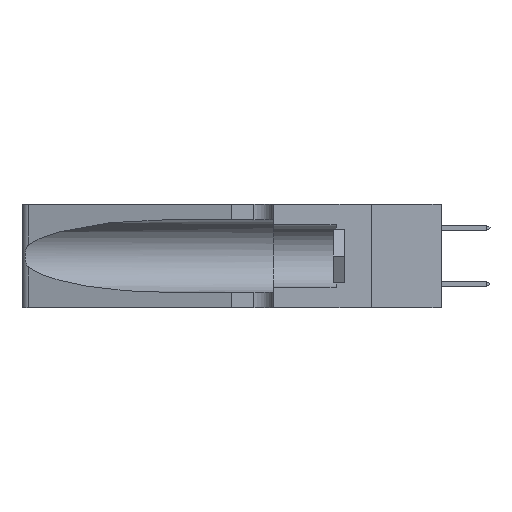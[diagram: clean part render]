
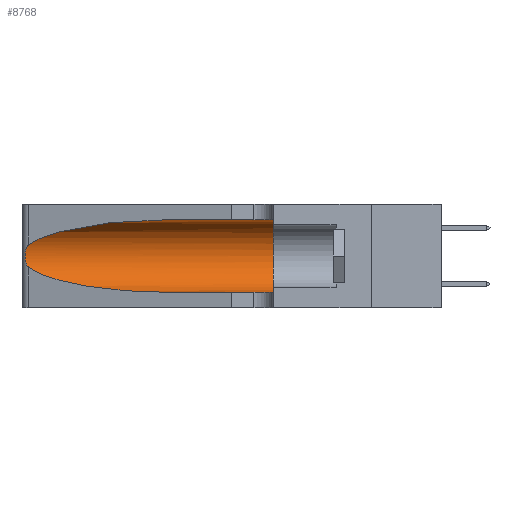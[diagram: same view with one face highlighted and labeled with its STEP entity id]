
A CAD part, left-side view. The second image highlights one B-rep face of the part: STEP entity #8768.
In plain terms, the highlighted cylindrical face has radius 3.308 mm (diameter 6.617 mm), a partial arc.
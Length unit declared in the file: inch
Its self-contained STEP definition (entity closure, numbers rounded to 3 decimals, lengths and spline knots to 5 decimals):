
#13 = LINE ( 'NONE', #13438, #5790 ) ;
#63 = ORIENTED_EDGE ( 'NONE', *, *, #6949, .F. ) ;
#84 =( BOUNDED_CURVE ( )  B_SPLINE_CURVE ( 3, ( #18097, #10203, #13347, #18655 ),
 .UNSPECIFIED., .F., .T. ) 
 B_SPLINE_CURVE_WITH_KNOTS ( ( 4, 4 ),
 ( 1.5708, 2.84003 ),
 .UNSPECIFIED. ) 
 CURVE ( )  GEOMETRIC_REPRESENTATION_ITEM ( )  RATIONAL_B_SPLINE_CURVE ( ( 1., 0.87, 0.87, 1. ) ) 
 REPRESENTATION_ITEM ( '' )  );
#110 = LINE ( 'NONE', #16641, #18577 ) ;
#367 = CARTESIAN_POINT ( 'NONE',  ( 0.25856, 1.23593, 0.16098 ) ) ;
#530 = DIRECTION ( 'NONE',  ( 0., -1., 0. ) ) ;
#2295 = ORIENTED_EDGE ( 'NONE', *, *, #19413, .F. ) ;
#2469 = DIRECTION ( 'NONE',  ( 0., 1., 0. ) ) ;
#3046 = CARTESIAN_POINT ( 'NONE',  ( 0.1305, 0.35, 0.31525 ) ) ;
#3513 = CARTESIAN_POINT ( 'NONE',  ( 0.25487, 1.22718, 0.14631 ) ) ;
#4180 = B_SPLINE_CURVE_WITH_KNOTS ( 'NONE', 3,
 ( #14332, #17677, #7968, #12981, #20914, #14555, #14627, #18074, #13321, #367, #13189, #14825, #16487, #3513 ),
 .UNSPECIFIED., .F., .F.,
 ( 4, 2, 2, 2, 2, 2, 4 ),
 ( 0., 0.00027, 0.00053, 0.00107, 0.0016, 0.00187, 0.00214 ),
 .UNSPECIFIED. ) ;
#4939 = CARTESIAN_POINT ( 'NONE',  ( 0.1305, 1.61858, 0.185 ) ) ;
#5483 = EDGE_CURVE ( 'NONE', #17042, #19116, #110, .T. ) ;
#5790 = VECTOR ( 'NONE', #15071, 39.37008 ) ;
#6294 = CARTESIAN_POINT ( 'NONE',  ( 0.1305, 0.72297, 0.31525 ) ) ;
#6671 = VERTEX_POINT ( 'NONE', #3046 ) ;
#6939 = CYLINDRICAL_SURFACE ( 'NONE', #7251, 0.13025 ) ;
#6949 = EDGE_CURVE ( 'NONE', #6671, #19116, #12541, .T. ) ;
#7251 = AXIS2_PLACEMENT_3D ( 'NONE', #4939, #9881, #14749 ) ;
#7319 =( BOUNDED_CURVE ( )  B_SPLINE_CURVE ( 3, ( #17235, #14317, #7516, #15929 ),
 .UNSPECIFIED., .F., .T. ) 
 B_SPLINE_CURVE_WITH_KNOTS ( ( 4, 4 ),
 ( 3.44316, 4.71239 ),
 .UNSPECIFIED. ) 
 CURVE ( )  GEOMETRIC_REPRESENTATION_ITEM ( )  RATIONAL_B_SPLINE_CURVE ( ( 1., 0.87, 0.87, 1. ) ) 
 REPRESENTATION_ITEM ( '' )  );
#7516 = CARTESIAN_POINT ( 'NONE',  ( 0.18966, 0.96281, 0.05475 ) ) ;
#7968 = CARTESIAN_POINT ( 'NONE',  ( 0.25639, 1.23184, 0.21858 ) ) ;
#8317 = CARTESIAN_POINT ( 'NONE',  ( 0.25487, 1.22718, 0.14631 ) ) ;
#8768 = ADVANCED_FACE ( 'NONE', ( #9777 ), #6939, .F. ) ;
#9203 = ORIENTED_EDGE ( 'NONE', *, *, #5483, .T. ) ;
#9473 = VERTEX_POINT ( 'NONE', #8317 ) ;
#9777 = FACE_OUTER_BOUND ( 'NONE', #10417, .T. ) ;
#9881 = DIRECTION ( 'NONE',  ( 0., -1., 0. ) ) ;
#10203 = CARTESIAN_POINT ( 'NONE',  ( 0.18966, 0.96281, 0.31525 ) ) ;
#10370 = ORIENTED_EDGE ( 'NONE', *, *, #19857, .T. ) ;
#10417 = EDGE_LOOP ( 'NONE', ( #17929, #10370, #15608, #9203, #63, #2295 ) ) ;
#10509 = EDGE_CURVE ( 'NONE', #19104, #12244, #84, .T. ) ;
#12244 = VERTEX_POINT ( 'NONE', #13776 ) ;
#12254 = CARTESIAN_POINT ( 'NONE',  ( 0.1305, 0.35, 0.185 ) ) ;
#12332 = DIRECTION ( 'NONE',  ( 0., 0., 1. ) ) ;
#12541 = CIRCLE ( 'NONE', #14993, 0.13025 ) ;
#12677 = EDGE_CURVE ( 'NONE', #9473, #17042, #7319, .T. ) ;
#12981 = CARTESIAN_POINT ( 'NONE',  ( 0.25787, 1.23484, 0.2124 ) ) ;
#13189 = CARTESIAN_POINT ( 'NONE',  ( 0.25789, 1.23486, 0.15765 ) ) ;
#13321 = CARTESIAN_POINT ( 'NONE',  ( 0.26017, 1.23833, 0.17102 ) ) ;
#13347 = CARTESIAN_POINT ( 'NONE',  ( 0.2373, 1.15595, 0.28018 ) ) ;
#13438 = CARTESIAN_POINT ( 'NONE',  ( 0.1305, 1.61858, 0.31525 ) ) ;
#13776 = CARTESIAN_POINT ( 'NONE',  ( 0.25487, 1.22718, 0.22369 ) ) ;
#14317 = CARTESIAN_POINT ( 'NONE',  ( 0.2373, 1.15595, 0.08982 ) ) ;
#14332 = CARTESIAN_POINT ( 'NONE',  ( 0.25487, 1.22718, 0.22369 ) ) ;
#14555 = CARTESIAN_POINT ( 'NONE',  ( 0.26018, 1.23835, 0.19895 ) ) ;
#14627 = CARTESIAN_POINT ( 'NONE',  ( 0.26075, 1.23896, 0.19203 ) ) ;
#14749 = DIRECTION ( 'NONE',  ( 0., 0., -1. ) ) ;
#14825 = CARTESIAN_POINT ( 'NONE',  ( 0.25639, 1.23186, 0.15144 ) ) ;
#14993 = AXIS2_PLACEMENT_3D ( 'NONE', #12254, #2469, #12332 ) ;
#15071 = DIRECTION ( 'NONE',  ( 0., -1., 0. ) ) ;
#15279 = CARTESIAN_POINT ( 'NONE',  ( 0.1305, 0.72297, 0.05475 ) ) ;
#15608 = ORIENTED_EDGE ( 'NONE', *, *, #12677, .T. ) ;
#15929 = CARTESIAN_POINT ( 'NONE',  ( 0.1305, 0.72297, 0.05475 ) ) ;
#16487 = CARTESIAN_POINT ( 'NONE',  ( 0.25555, 1.22993, 0.14849 ) ) ;
#16641 = CARTESIAN_POINT ( 'NONE',  ( 0.1305, 1.61858, 0.05475 ) ) ;
#17042 = VERTEX_POINT ( 'NONE', #15279 ) ;
#17235 = CARTESIAN_POINT ( 'NONE',  ( 0.25487, 1.22718, 0.14631 ) ) ;
#17655 = CARTESIAN_POINT ( 'NONE',  ( 0.1305, 0.35, 0.05475 ) ) ;
#17677 = CARTESIAN_POINT ( 'NONE',  ( 0.25555, 1.22994, 0.2215 ) ) ;
#17929 = ORIENTED_EDGE ( 'NONE', *, *, #10509, .T. ) ;
#18074 = CARTESIAN_POINT ( 'NONE',  ( 0.26075, 1.23896, 0.178 ) ) ;
#18097 = CARTESIAN_POINT ( 'NONE',  ( 0.1305, 0.72297, 0.31525 ) ) ;
#18577 = VECTOR ( 'NONE', #530, 39.37008 ) ;
#18655 = CARTESIAN_POINT ( 'NONE',  ( 0.25487, 1.22718, 0.22369 ) ) ;
#19104 = VERTEX_POINT ( 'NONE', #6294 ) ;
#19116 = VERTEX_POINT ( 'NONE', #17655 ) ;
#19413 = EDGE_CURVE ( 'NONE', #19104, #6671, #13, .T. ) ;
#19857 = EDGE_CURVE ( 'NONE', #12244, #9473, #4180, .T. ) ;
#20914 = CARTESIAN_POINT ( 'NONE',  ( 0.25854, 1.2359, 0.20912 ) ) ;
